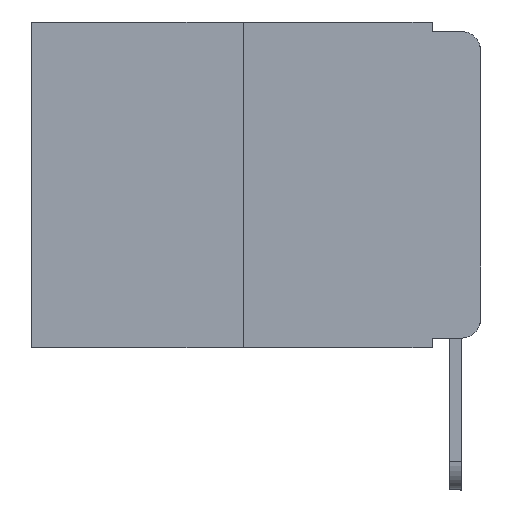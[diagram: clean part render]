
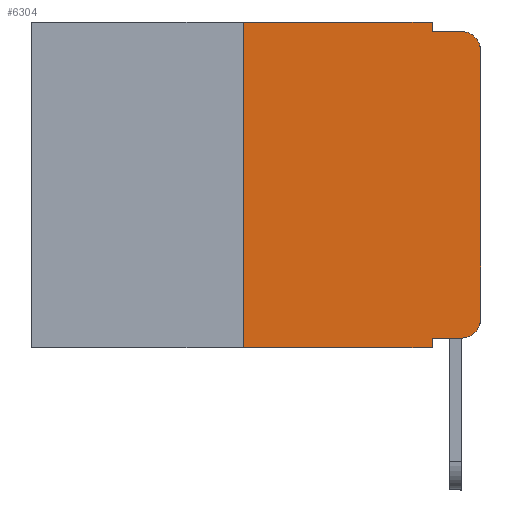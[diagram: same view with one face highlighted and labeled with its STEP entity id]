
A CAD part, left-side view. The second image highlights one B-rep face of the part: STEP entity #6304.
In plain terms, the highlighted planar face has unit normal (-1, 0, 0).
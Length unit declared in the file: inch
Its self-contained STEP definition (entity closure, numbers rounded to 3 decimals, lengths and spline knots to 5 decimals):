
#85 = CARTESIAN_POINT ( 'NONE',  ( 0., 0.051, 0. ) ) ;
#117 = CARTESIAN_POINT ( 'NONE',  ( 0., 0.25, -0.343 ) ) ;
#119 = CARTESIAN_POINT ( 'NONE',  ( 0., 0.02, -0.01 ) ) ;
#331 = AXIS2_PLACEMENT_3D ( 'NONE', #14307, #9618, #19714 ) ;
#378 = DIRECTION ( 'NONE',  ( 0., -1., 0. ) ) ;
#524 = ORIENTED_EDGE ( 'NONE', *, *, #9331, .T. ) ;
#738 = EDGE_CURVE ( 'NONE', #17687, #15260, #16666, .T. ) ;
#813 = DIRECTION ( 'NONE',  ( 0., 0., -1. ) ) ;
#1010 = VERTEX_POINT ( 'NONE', #8223 ) ;
#1365 = ORIENTED_EDGE ( 'NONE', *, *, #2735, .T. ) ;
#1402 = DIRECTION ( 'NONE',  ( -1., 0., 0. ) ) ;
#1993 = ORIENTED_EDGE ( 'NONE', *, *, #8154, .F. ) ;
#2035 = DIRECTION ( 'NONE',  ( 0., 0., -1. ) ) ;
#2266 = VERTEX_POINT ( 'NONE', #85 ) ;
#2735 = EDGE_CURVE ( 'NONE', #16100, #10726, #16820, .T. ) ;
#3707 = CARTESIAN_POINT ( 'NONE',  ( 0., 0.051, -0.01 ) ) ;
#3750 = EDGE_CURVE ( 'NONE', #1010, #4767, #18218, .T. ) ;
#3921 = AXIS2_PLACEMENT_3D ( 'NONE', #11134, #1402, #4945 ) ;
#3980 = CARTESIAN_POINT ( 'NONE',  ( 0., 0., 0. ) ) ;
#4068 = ORIENTED_EDGE ( 'NONE', *, *, #11818, .F. ) ;
#4542 = CARTESIAN_POINT ( 'NONE',  ( 0., 0., -0.313 ) ) ;
#4767 = VERTEX_POINT ( 'NONE', #119 ) ;
#4945 = DIRECTION ( 'NONE',  ( 0., 0., -1. ) ) ;
#5024 = LINE ( 'NONE', #9751, #17297 ) ;
#5040 = ORIENTED_EDGE ( 'NONE', *, *, #18826, .T. ) ;
#5061 = ORIENTED_EDGE ( 'NONE', *, *, #6259, .F. ) ;
#5332 = DIRECTION ( 'NONE',  ( 0., 0., 1. ) ) ;
#5747 = LINE ( 'NONE', #14866, #6103 ) ;
#5885 = VERTEX_POINT ( 'NONE', #16368 ) ;
#6103 = VECTOR ( 'NONE', #12053, 39.37008 ) ;
#6259 = EDGE_CURVE ( 'NONE', #5885, #4767, #17706, .T. ) ;
#6304 = ADVANCED_FACE ( 'NONE', ( #8045 ), #13010, .F. ) ;
#6389 = ORIENTED_EDGE ( 'NONE', *, *, #738, .T. ) ;
#6501 = DIRECTION ( 'NONE',  ( 0., -1., 0. ) ) ;
#6602 = CARTESIAN_POINT ( 'NONE',  ( 0., 0.473, 0. ) ) ;
#6652 = CARTESIAN_POINT ( 'NONE',  ( 0., 0.02, -0.333 ) ) ;
#6736 = VERTEX_POINT ( 'NONE', #9866 ) ;
#6802 = AXIS2_PLACEMENT_3D ( 'NONE', #6602, #13216, #2035 ) ;
#7129 = VECTOR ( 'NONE', #378, 39.37008 ) ;
#7213 = DIRECTION ( 'NONE',  ( 0., -1., 0. ) ) ;
#7402 = ORIENTED_EDGE ( 'NONE', *, *, #14846, .F. ) ;
#7763 = VECTOR ( 'NONE', #5332, 39.37008 ) ;
#8045 = FACE_OUTER_BOUND ( 'NONE', #10929, .T. ) ;
#8154 = EDGE_CURVE ( 'NONE', #10483, #15260, #5747, .T. ) ;
#8223 = CARTESIAN_POINT ( 'NONE',  ( 0., 0., -0.03 ) ) ;
#9331 = EDGE_CURVE ( 'NONE', #10483, #16100, #13331, .T. ) ;
#9618 = DIRECTION ( 'NONE',  ( -1., 0., 0. ) ) ;
#9751 = CARTESIAN_POINT ( 'NONE',  ( 0., 0.25, 0. ) ) ;
#9866 = CARTESIAN_POINT ( 'NONE',  ( 0., 0.25, 0. ) ) ;
#9925 = CARTESIAN_POINT ( 'NONE',  ( 0., 0.051, -0.343 ) ) ;
#10483 = VERTEX_POINT ( 'NONE', #13441 ) ;
#10726 = VERTEX_POINT ( 'NONE', #4542 ) ;
#10929 = EDGE_LOOP ( 'NONE', ( #5040, #18403, #5061, #4068, #13849, #7402, #6389, #1993, #524, #1365 ) ) ;
#11134 = CARTESIAN_POINT ( 'NONE',  ( 0., 0.02, -0.313 ) ) ;
#11508 = VECTOR ( 'NONE', #11676, 39.37008 ) ;
#11676 = DIRECTION ( 'NONE',  ( 0., -1., 0. ) ) ;
#11818 = EDGE_CURVE ( 'NONE', #2266, #5885, #18131, .T. ) ;
#12053 = DIRECTION ( 'NONE',  ( 0., 0., -1. ) ) ;
#12801 = CARTESIAN_POINT ( 'NONE',  ( 0., 0.473, 0. ) ) ;
#13010 = PLANE ( 'NONE',  #6802 ) ;
#13216 = DIRECTION ( 'NONE',  ( 1., 0., 0. ) ) ;
#13331 = LINE ( 'NONE', #16551, #11508 ) ;
#13441 = CARTESIAN_POINT ( 'NONE',  ( 0., 0.051, -0.333 ) ) ;
#13849 = ORIENTED_EDGE ( 'NONE', *, *, #19444, .F. ) ;
#14204 = VECTOR ( 'NONE', #813, 39.37008 ) ;
#14307 = CARTESIAN_POINT ( 'NONE',  ( 0., 0.02, -0.03 ) ) ;
#14332 = VECTOR ( 'NONE', #7213, 39.37008 ) ;
#14846 = EDGE_CURVE ( 'NONE', #17687, #6736, #5024, .T. ) ;
#14866 = CARTESIAN_POINT ( 'NONE',  ( 0., 0.051, 0. ) ) ;
#15260 = VERTEX_POINT ( 'NONE', #9925 ) ;
#16075 = VECTOR ( 'NONE', #6501, 39.37008 ) ;
#16100 = VERTEX_POINT ( 'NONE', #6652 ) ;
#16200 = LINE ( 'NONE', #3980, #7763 ) ;
#16368 = CARTESIAN_POINT ( 'NONE',  ( 0., 0.051, -0.01 ) ) ;
#16551 = CARTESIAN_POINT ( 'NONE',  ( 0., 0.051, -0.333 ) ) ;
#16666 = LINE ( 'NONE', #16766, #14332 ) ;
#16766 = CARTESIAN_POINT ( 'NONE',  ( 0., 0.473, -0.343 ) ) ;
#16820 = CIRCLE ( 'NONE', #3921, 0.02 ) ;
#17297 = VECTOR ( 'NONE', #19206, 39.37008 ) ;
#17598 = LINE ( 'NONE', #12801, #7129 ) ;
#17687 = VERTEX_POINT ( 'NONE', #117 ) ;
#17706 = LINE ( 'NONE', #3707, #16075 ) ;
#18131 = LINE ( 'NONE', #18335, #14204 ) ;
#18218 = CIRCLE ( 'NONE', #331, 0.02 ) ;
#18335 = CARTESIAN_POINT ( 'NONE',  ( 0., 0.051, 0. ) ) ;
#18403 = ORIENTED_EDGE ( 'NONE', *, *, #3750, .T. ) ;
#18826 = EDGE_CURVE ( 'NONE', #10726, #1010, #16200, .T. ) ;
#19206 = DIRECTION ( 'NONE',  ( 0., 0., 1. ) ) ;
#19444 = EDGE_CURVE ( 'NONE', #6736, #2266, #17598, .T. ) ;
#19714 = DIRECTION ( 'NONE',  ( 0., 0., -1. ) ) ;
